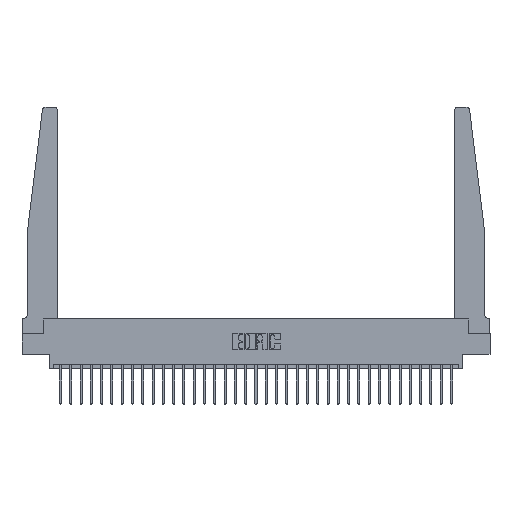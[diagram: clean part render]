
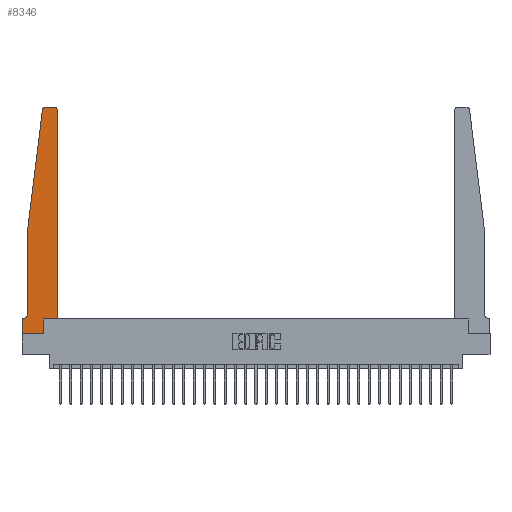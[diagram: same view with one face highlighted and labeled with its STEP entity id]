
A CAD part, top view. The second image highlights one B-rep face of the part: STEP entity #8346.
In plain terms, the highlighted planar face has unit normal (0, 0, 1).
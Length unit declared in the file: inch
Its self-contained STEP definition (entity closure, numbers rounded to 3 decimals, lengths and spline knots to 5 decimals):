
#268 = AXIS2_PLACEMENT_3D ( 'NONE', #19506, #21924, #7642 ) ;
#606 = CARTESIAN_POINT ( 'NONE',  ( 0.27653, 2.75, 0.37 ) ) ;
#786 = CIRCLE ( 'NONE', #18005, 0.03 ) ;
#847 = DIRECTION ( 'NONE',  ( 0., 0., 1. ) ) ;
#859 = VECTOR ( 'NONE', #20130, 39.37008 ) ;
#1426 = ORIENTED_EDGE ( 'NONE', *, *, #15529, .T. ) ;
#1448 = VERTEX_POINT ( 'NONE', #17185 ) ;
#1616 = LINE ( 'NONE', #5874, #859 ) ;
#2286 = LINE ( 'NONE', #2652, #7861 ) ;
#2438 = EDGE_CURVE ( 'NONE', #23364, #28675, #1616, .T. ) ;
#2520 = CARTESIAN_POINT ( 'NONE',  ( 0.015, 0.1875, 0.37 ) ) ;
#2652 = CARTESIAN_POINT ( 'NONE',  ( 0.25, 2.75, 0.37 ) ) ;
#2868 = PLANE ( 'NONE',  #268 ) ;
#3516 = VECTOR ( 'NONE', #24025, 39.37008 ) ;
#4002 = DIRECTION ( 'NONE',  ( 0., -1., 0. ) ) ;
#5025 = LINE ( 'NONE', #25585, #23242 ) ;
#5368 = CARTESIAN_POINT ( 'NONE',  ( 0.425, 0.18, 0.37 ) ) ;
#5472 = CIRCLE ( 'NONE', #14389, 0.03 ) ;
#5633 = CARTESIAN_POINT ( 'NONE',  ( 0.065, 1.25, 0.37 ) ) ;
#5874 = CARTESIAN_POINT ( 'NONE',  ( 0.065, 0.1875, 0.37 ) ) ;
#6019 = CARTESIAN_POINT ( 'NONE',  ( 0.425, 0.18, 0.37 ) ) ;
#6145 = CARTESIAN_POINT ( 'NONE',  ( 0.2605, 0., 0.37 ) ) ;
#6436 = LINE ( 'NONE', #25059, #18323 ) ;
#6716 = CARTESIAN_POINT ( 'NONE',  ( 0., 0., 0.37 ) ) ;
#6742 = CARTESIAN_POINT ( 'NONE',  ( 0., 0., 0.37 ) ) ;
#6956 = VERTEX_POINT ( 'NONE', #606 ) ;
#7350 = CARTESIAN_POINT ( 'NONE',  ( 0.065, 1.25, 0.37 ) ) ;
#7486 = CARTESIAN_POINT ( 'NONE',  ( 0.425, 0.18, 0.37 ) ) ;
#7642 = DIRECTION ( 'NONE',  ( 1., 0., 0. ) ) ;
#7861 = VECTOR ( 'NONE', #12106, 39.37008 ) ;
#8320 = ORIENTED_EDGE ( 'NONE', *, *, #2438, .T. ) ;
#8346 = ADVANCED_FACE ( 'NONE', ( #28602 ), #2868, .T. ) ;
#8873 = ORIENTED_EDGE ( 'NONE', *, *, #28252, .T. ) ;
#9518 = EDGE_CURVE ( 'NONE', #17536, #1448, #17692, .T. ) ;
#9733 = EDGE_CURVE ( 'NONE', #22544, #17536, #21839, .T. ) ;
#9886 = AXIS2_PLACEMENT_3D ( 'NONE', #24459, #10146, #26824 ) ;
#10146 = DIRECTION ( 'NONE',  ( 0., 0., -1. ) ) ;
#10379 = CARTESIAN_POINT ( 'NONE',  ( 0.395, 2.75, 0.37 ) ) ;
#10516 = EDGE_CURVE ( 'NONE', #12808, #22544, #5025, .T. ) ;
#10732 = VERTEX_POINT ( 'NONE', #12393 ) ;
#11510 = VERTEX_POINT ( 'NONE', #10379 ) ;
#11911 = ORIENTED_EDGE ( 'NONE', *, *, #9518, .T. ) ;
#12106 = DIRECTION ( 'NONE',  ( -1., 0., 0. ) ) ;
#12268 = EDGE_CURVE ( 'NONE', #23591, #20371, #15352, .T. ) ;
#12393 = CARTESIAN_POINT ( 'NONE',  ( 0.24675, 2.72367, 0.37 ) ) ;
#12808 = VERTEX_POINT ( 'NONE', #6145 ) ;
#13040 = DIRECTION ( 'NONE',  ( 1., 0., 0. ) ) ;
#13796 = CARTESIAN_POINT ( 'NONE',  ( 0.395, 2.72, 0.37 ) ) ;
#14389 = AXIS2_PLACEMENT_3D ( 'NONE', #13796, #30422, #16188 ) ;
#14502 = ORIENTED_EDGE ( 'NONE', *, *, #25390, .T. ) ;
#15112 = CARTESIAN_POINT ( 'NONE',  ( 0.27653, 2.72, 0.37 ) ) ;
#15352 = LINE ( 'NONE', #15924, #22446 ) ;
#15529 = EDGE_CURVE ( 'NONE', #28675, #20419, #19912, .T. ) ;
#15699 = EDGE_CURVE ( 'NONE', #10732, #23591, #16153, .T. ) ;
#15924 = CARTESIAN_POINT ( 'NONE',  ( 0.065, 1.25, 0.37 ) ) ;
#16153 = LINE ( 'NONE', #7350, #3516 ) ;
#16188 = DIRECTION ( 'NONE',  ( 1., 0., 0. ) ) ;
#16540 = CARTESIAN_POINT ( 'NONE',  ( 0., 0.1875, 0.37 ) ) ;
#17185 = CARTESIAN_POINT ( 'NONE',  ( 0.425, 2.72, 0.37 ) ) ;
#17453 = EDGE_CURVE ( 'NONE', #11510, #6956, #2286, .T. ) ;
#17470 = DIRECTION ( 'NONE',  ( 1., 0., 0. ) ) ;
#17536 = VERTEX_POINT ( 'NONE', #5368 ) ;
#17692 = LINE ( 'NONE', #7486, #30352 ) ;
#18005 = AXIS2_PLACEMENT_3D ( 'NONE', #15112, #847, #17470 ) ;
#18253 = CIRCLE ( 'NONE', #9886, 0.05 ) ;
#18323 = VECTOR ( 'NONE', #13040, 39.37008 ) ;
#19506 = CARTESIAN_POINT ( 'NONE',  ( 0., 0.1875, 0.37 ) ) ;
#19529 = ORIENTED_EDGE ( 'NONE', *, *, #12268, .T. ) ;
#19912 = LINE ( 'NONE', #6742, #25535 ) ;
#20130 = DIRECTION ( 'NONE',  ( -1., 0., 0. ) ) ;
#20371 = VERTEX_POINT ( 'NONE', #20778 ) ;
#20419 = VERTEX_POINT ( 'NONE', #6716 ) ;
#20755 = DIRECTION ( 'NONE',  ( 0., 1., 0. ) ) ;
#20778 = CARTESIAN_POINT ( 'NONE',  ( 0.065, 0.2375, 0.37 ) ) ;
#20931 = EDGE_CURVE ( 'NONE', #20419, #12808, #6436, .T. ) ;
#21429 = ORIENTED_EDGE ( 'NONE', *, *, #15699, .T. ) ;
#21839 = LINE ( 'NONE', #6019, #25209 ) ;
#21924 = DIRECTION ( 'NONE',  ( 0., 0., 1. ) ) ;
#22395 = EDGE_LOOP ( 'NONE', ( #24450, #8873, #21429, #19529, #24406, #8320, #1426, #23440, #22682, #28431, #11911, #14502 ) ) ;
#22446 = VECTOR ( 'NONE', #4002, 39.37008 ) ;
#22544 = VERTEX_POINT ( 'NONE', #29914 ) ;
#22664 = DIRECTION ( 'NONE',  ( 1., 0., 0. ) ) ;
#22682 = ORIENTED_EDGE ( 'NONE', *, *, #10516, .T. ) ;
#23242 = VECTOR ( 'NONE', #20755, 39.37008 ) ;
#23364 = VERTEX_POINT ( 'NONE', #2520 ) ;
#23440 = ORIENTED_EDGE ( 'NONE', *, *, #20931, .T. ) ;
#23591 = VERTEX_POINT ( 'NONE', #5633 ) ;
#24025 = DIRECTION ( 'NONE',  ( -0.122, -0.992, 0. ) ) ;
#24168 = DIRECTION ( 'NONE',  ( 0., 1., 0. ) ) ;
#24406 = ORIENTED_EDGE ( 'NONE', *, *, #29481, .T. ) ;
#24450 = ORIENTED_EDGE ( 'NONE', *, *, #17453, .T. ) ;
#24459 = CARTESIAN_POINT ( 'NONE',  ( 0.015, 0.2375, 0.37 ) ) ;
#25059 = CARTESIAN_POINT ( 'NONE',  ( 0., 0., 0.37 ) ) ;
#25209 = VECTOR ( 'NONE', #22664, 39.37008 ) ;
#25390 = EDGE_CURVE ( 'NONE', #1448, #11510, #5472, .T. ) ;
#25535 = VECTOR ( 'NONE', #25841, 39.37008 ) ;
#25585 = CARTESIAN_POINT ( 'NONE',  ( 0.2605, 0.18, 0.37 ) ) ;
#25841 = DIRECTION ( 'NONE',  ( 0., -1., 0. ) ) ;
#26824 = DIRECTION ( 'NONE',  ( -1., 0., 0. ) ) ;
#28252 = EDGE_CURVE ( 'NONE', #6956, #10732, #786, .T. ) ;
#28431 = ORIENTED_EDGE ( 'NONE', *, *, #9733, .T. ) ;
#28602 = FACE_OUTER_BOUND ( 'NONE', #22395, .T. ) ;
#28675 = VERTEX_POINT ( 'NONE', #16540 ) ;
#29481 = EDGE_CURVE ( 'NONE', #20371, #23364, #18253, .T. ) ;
#29914 = CARTESIAN_POINT ( 'NONE',  ( 0.2605, 0.18, 0.37 ) ) ;
#30352 = VECTOR ( 'NONE', #24168, 39.37008 ) ;
#30422 = DIRECTION ( 'NONE',  ( 0., 0., 1. ) ) ;
